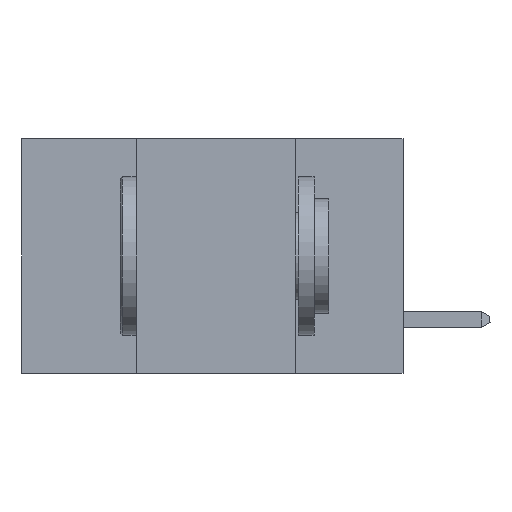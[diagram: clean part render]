
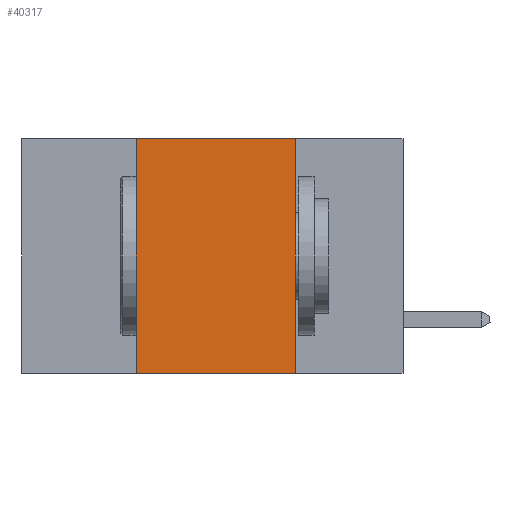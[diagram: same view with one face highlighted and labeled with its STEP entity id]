
A CAD part, left-side view. The second image highlights one B-rep face of the part: STEP entity #40317.
In plain terms, the highlighted planar face has unit normal (-1, 0, 0).
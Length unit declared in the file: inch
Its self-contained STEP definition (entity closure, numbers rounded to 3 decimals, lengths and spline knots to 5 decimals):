
#88 = LINE ( 'NONE', #25417, #18244 ) ;
#2410 = CARTESIAN_POINT ( 'NONE',  ( 0., 0.6, 0. ) ) ;
#2424 = VECTOR ( 'NONE', #33709, 39.37008 ) ;
#2863 = LINE ( 'NONE', #5465, #11824 ) ;
#3079 = LINE ( 'NONE', #14201, #9020 ) ;
#4918 = EDGE_CURVE ( 'NONE', #11124, #23574, #3079, .T. ) ;
#5465 = CARTESIAN_POINT ( 'NONE',  ( 0., 0.17, 0. ) ) ;
#5537 = CARTESIAN_POINT ( 'NONE',  ( 0., 0.17, -0.37 ) ) ;
#7485 = CARTESIAN_POINT ( 'NONE',  ( 0., 0.42, 0. ) ) ;
#8455 = FACE_OUTER_BOUND ( 'NONE', #36134, .T. ) ;
#9020 = VECTOR ( 'NONE', #36802, 39.37008 ) ;
#9942 = AXIS2_PLACEMENT_3D ( 'NONE', #2410, #11904, #28419 ) ;
#10772 = VERTEX_POINT ( 'NONE', #40616 ) ;
#11124 = VERTEX_POINT ( 'NONE', #12209 ) ;
#11824 = VECTOR ( 'NONE', #12015, 39.37008 ) ;
#11904 = DIRECTION ( 'NONE',  ( 1., 0., 0. ) ) ;
#12015 = DIRECTION ( 'NONE',  ( 0., 0., -1. ) ) ;
#12209 = CARTESIAN_POINT ( 'NONE',  ( 0., 0.42, -0.37 ) ) ;
#14201 = CARTESIAN_POINT ( 'NONE',  ( 0., 0.6, -0.37 ) ) ;
#14654 = ORIENTED_EDGE ( 'NONE', *, *, #26646, .F. ) ;
#18244 = VECTOR ( 'NONE', #18864, 39.37008 ) ;
#18864 = DIRECTION ( 'NONE',  ( 0., -1., 0. ) ) ;
#23574 = VERTEX_POINT ( 'NONE', #5537 ) ;
#25044 = LINE ( 'NONE', #7485, #2424 ) ;
#25417 = CARTESIAN_POINT ( 'NONE',  ( 0., 0.6, 0. ) ) ;
#26646 = EDGE_CURVE ( 'NONE', #34439, #23574, #2863, .T. ) ;
#27835 = PLANE ( 'NONE',  #9942 ) ;
#28419 = DIRECTION ( 'NONE',  ( 0., 0., -1. ) ) ;
#28693 = ORIENTED_EDGE ( 'NONE', *, *, #4918, .T. ) ;
#30710 = ORIENTED_EDGE ( 'NONE', *, *, #40779, .F. ) ;
#33709 = DIRECTION ( 'NONE',  ( 0., 0., 1. ) ) ;
#34439 = VERTEX_POINT ( 'NONE', #40828 ) ;
#36134 = EDGE_LOOP ( 'NONE', ( #14654, #38016, #30710, #28693 ) ) ;
#36802 = DIRECTION ( 'NONE',  ( 0., -1., 0. ) ) ;
#38016 = ORIENTED_EDGE ( 'NONE', *, *, #38535, .F. ) ;
#38535 = EDGE_CURVE ( 'NONE', #10772, #34439, #88, .T. ) ;
#40317 = ADVANCED_FACE ( 'NONE', ( #8455 ), #27835, .F. ) ;
#40616 = CARTESIAN_POINT ( 'NONE',  ( 0., 0.42, 0. ) ) ;
#40779 = EDGE_CURVE ( 'NONE', #11124, #10772, #25044, .T. ) ;
#40828 = CARTESIAN_POINT ( 'NONE',  ( 0., 0.17, 0. ) ) ;
